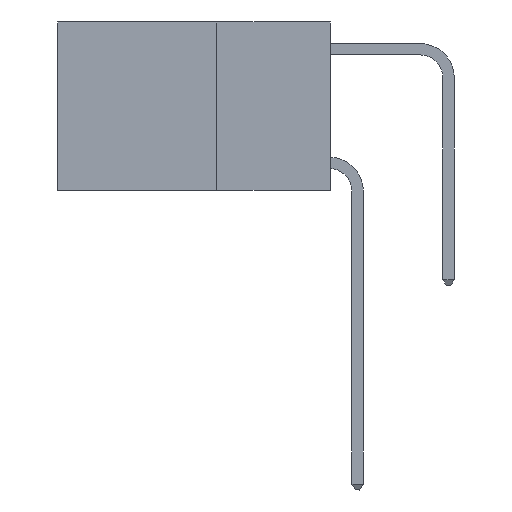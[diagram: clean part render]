
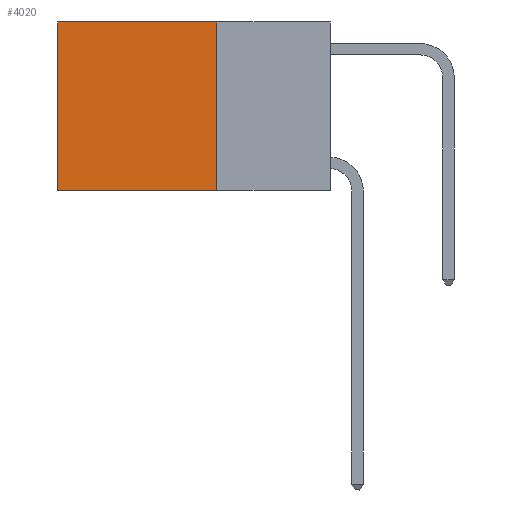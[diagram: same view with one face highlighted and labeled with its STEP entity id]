
A CAD part, left-side view. The second image highlights one B-rep face of the part: STEP entity #4020.
In plain terms, the highlighted planar face has unit normal (-1, 0, 0).
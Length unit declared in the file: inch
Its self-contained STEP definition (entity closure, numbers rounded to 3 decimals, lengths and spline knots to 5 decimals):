
#297 = CARTESIAN_POINT ( 'NONE',  ( 0.2625, 0.6, -0.37 ) ) ;
#756 = CARTESIAN_POINT ( 'NONE',  ( 0.2625, 0.25, 0. ) ) ;
#955 = PLANE ( 'NONE',  #12710 ) ;
#1005 = VECTOR ( 'NONE', #17411, 39.37008 ) ;
#1071 = CARTESIAN_POINT ( 'NONE',  ( 0.2625, 0.25, 0. ) ) ;
#2014 = VECTOR ( 'NONE', #9198, 39.37008 ) ;
#2987 = CARTESIAN_POINT ( 'NONE',  ( 0.2625, 0.25, 0. ) ) ;
#4020 = ADVANCED_FACE ( 'NONE', ( #16024 ), #955, .F. ) ;
#4677 = EDGE_CURVE ( 'NONE', #11210, #6151, #8420, .T. ) ;
#4680 = LINE ( 'NONE', #756, #1005 ) ;
#4847 = EDGE_CURVE ( 'NONE', #12199, #9304, #13390, .T. ) ;
#6151 = VERTEX_POINT ( 'NONE', #297 ) ;
#6967 = CARTESIAN_POINT ( 'NONE',  ( 0.2625, 0.6, 0. ) ) ;
#7482 = CARTESIAN_POINT ( 'NONE',  ( 0.2625, 0.25, 0. ) ) ;
#7641 = CARTESIAN_POINT ( 'NONE',  ( 0.2625, 0.25, -0.37 ) ) ;
#7693 = CARTESIAN_POINT ( 'NONE',  ( 0.2625, 0.25, -0.37 ) ) ;
#7854 = DIRECTION ( 'NONE',  ( 1., 0., 0. ) ) ;
#8420 = LINE ( 'NONE', #7693, #2014 ) ;
#9198 = DIRECTION ( 'NONE',  ( 0., 1., 0. ) ) ;
#9304 = VERTEX_POINT ( 'NONE', #6967 ) ;
#10540 = DIRECTION ( 'NONE',  ( 0., 0., -1. ) ) ;
#11210 = VERTEX_POINT ( 'NONE', #7641 ) ;
#11735 = ORIENTED_EDGE ( 'NONE', *, *, #14393, .T. ) ;
#12199 = VERTEX_POINT ( 'NONE', #2987 ) ;
#12710 = AXIS2_PLACEMENT_3D ( 'NONE', #1071, #7854, #10540 ) ;
#13249 = VECTOR ( 'NONE', #14214, 39.37008 ) ;
#13390 = LINE ( 'NONE', #7482, #14036 ) ;
#13996 = EDGE_CURVE ( 'NONE', #12199, #11210, #4680, .T. ) ;
#14036 = VECTOR ( 'NONE', #15911, 39.37008 ) ;
#14214 = DIRECTION ( 'NONE',  ( 0., 0., -1. ) ) ;
#14393 = EDGE_CURVE ( 'NONE', #9304, #6151, #15003, .T. ) ;
#15003 = LINE ( 'NONE', #15506, #13249 ) ;
#15506 = CARTESIAN_POINT ( 'NONE',  ( 0.2625, 0.6, 0. ) ) ;
#15911 = DIRECTION ( 'NONE',  ( 0., 1., 0. ) ) ;
#16024 = FACE_OUTER_BOUND ( 'NONE', #16190, .T. ) ;
#16190 = EDGE_LOOP ( 'NONE', ( #11735, #17504, #16963, #16332 ) ) ;
#16332 = ORIENTED_EDGE ( 'NONE', *, *, #4847, .T. ) ;
#16963 = ORIENTED_EDGE ( 'NONE', *, *, #13996, .F. ) ;
#17411 = DIRECTION ( 'NONE',  ( 0., 0., -1. ) ) ;
#17504 = ORIENTED_EDGE ( 'NONE', *, *, #4677, .F. ) ;
